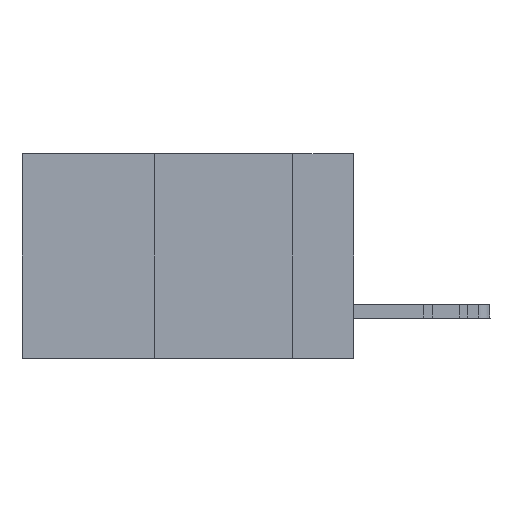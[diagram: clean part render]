
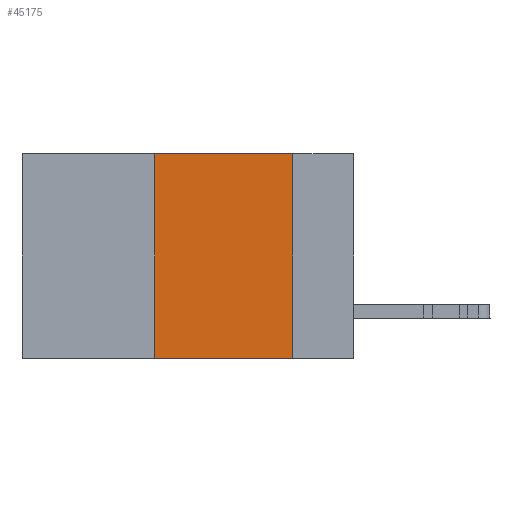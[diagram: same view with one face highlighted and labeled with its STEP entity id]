
A CAD part, left-side view. The second image highlights one B-rep face of the part: STEP entity #45175.
In plain terms, the highlighted planar face has unit normal (-1, 0, 0).
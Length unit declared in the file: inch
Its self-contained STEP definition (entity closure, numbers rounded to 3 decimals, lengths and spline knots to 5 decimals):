
#287 = CARTESIAN_POINT ( 'NONE',  ( 0., 0.6, 0. ) ) ;
#1480 = EDGE_CURVE ( 'NONE', #20313, #43246, #22336, .T. ) ;
#4227 = EDGE_CURVE ( 'NONE', #44993, #20313, #44940, .T. ) ;
#5009 = DIRECTION ( 'NONE',  ( 0., 0., -1. ) ) ;
#5102 = ORIENTED_EDGE ( 'NONE', *, *, #4227, .F. ) ;
#9320 = DIRECTION ( 'NONE',  ( 1., 0., 0. ) ) ;
#10041 = AXIS2_PLACEMENT_3D ( 'NONE', #31062, #9320, #5009 ) ;
#10786 = VECTOR ( 'NONE', #14615, 39.37008 ) ;
#11134 = FACE_OUTER_BOUND ( 'NONE', #43874, .T. ) ;
#13358 = VECTOR ( 'NONE', #45623, 39.37008 ) ;
#14212 = LINE ( 'NONE', #14767, #10786 ) ;
#14615 = DIRECTION ( 'NONE',  ( 0., 0., -1. ) ) ;
#14767 = CARTESIAN_POINT ( 'NONE',  ( 0., 0.11, 0. ) ) ;
#18566 = DIRECTION ( 'NONE',  ( 0., -1., 0. ) ) ;
#18841 = VERTEX_POINT ( 'NONE', #43748 ) ;
#19469 = CARTESIAN_POINT ( 'NONE',  ( 0., 0.36, 0. ) ) ;
#20313 = VERTEX_POINT ( 'NONE', #46923 ) ;
#21929 = ORIENTED_EDGE ( 'NONE', *, *, #41344, .T. ) ;
#22336 = LINE ( 'NONE', #287, #29793 ) ;
#22911 = ORIENTED_EDGE ( 'NONE', *, *, #1480, .F. ) ;
#24455 = VECTOR ( 'NONE', #26873, 39.37008 ) ;
#26873 = DIRECTION ( 'NONE',  ( 0., 0., 1. ) ) ;
#28749 = LINE ( 'NONE', #31413, #13358 ) ;
#29793 = VECTOR ( 'NONE', #18566, 39.37008 ) ;
#31062 = CARTESIAN_POINT ( 'NONE',  ( 0., 0.6, 0. ) ) ;
#31413 = CARTESIAN_POINT ( 'NONE',  ( 0., 0.6, -0.37 ) ) ;
#34077 = PLANE ( 'NONE',  #10041 ) ;
#39790 = EDGE_CURVE ( 'NONE', #43246, #18841, #14212, .T. ) ;
#41344 = EDGE_CURVE ( 'NONE', #44993, #18841, #28749, .T. ) ;
#43246 = VERTEX_POINT ( 'NONE', #43339 ) ;
#43339 = CARTESIAN_POINT ( 'NONE',  ( 0., 0.11, 0. ) ) ;
#43748 = CARTESIAN_POINT ( 'NONE',  ( 0., 0.11, -0.37 ) ) ;
#43874 = EDGE_LOOP ( 'NONE', ( #46734, #22911, #5102, #21929 ) ) ;
#44325 = CARTESIAN_POINT ( 'NONE',  ( 0., 0.36, -0.37 ) ) ;
#44940 = LINE ( 'NONE', #19469, #24455 ) ;
#44993 = VERTEX_POINT ( 'NONE', #44325 ) ;
#45175 = ADVANCED_FACE ( 'NONE', ( #11134 ), #34077, .F. ) ;
#45623 = DIRECTION ( 'NONE',  ( 0., -1., 0. ) ) ;
#46734 = ORIENTED_EDGE ( 'NONE', *, *, #39790, .F. ) ;
#46923 = CARTESIAN_POINT ( 'NONE',  ( 0., 0.36, 0. ) ) ;
